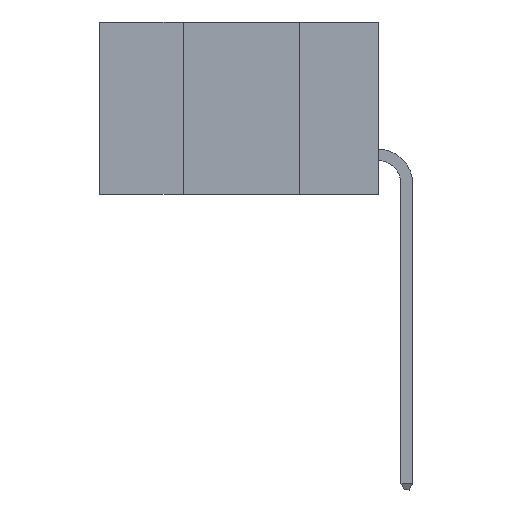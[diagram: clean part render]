
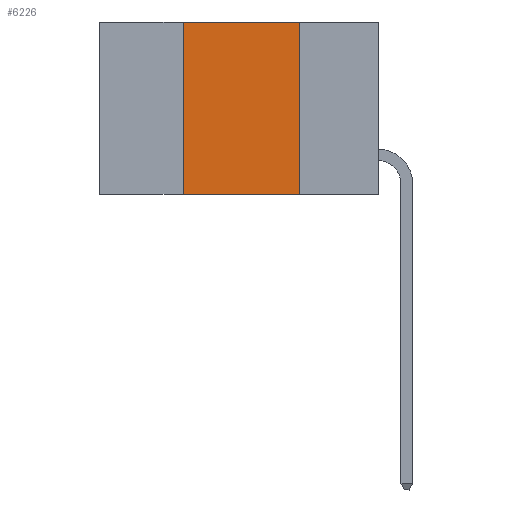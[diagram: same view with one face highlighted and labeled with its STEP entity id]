
A CAD part, left-side view. The second image highlights one B-rep face of the part: STEP entity #6226.
In plain terms, the highlighted planar face has unit normal (-1, 0, 0).
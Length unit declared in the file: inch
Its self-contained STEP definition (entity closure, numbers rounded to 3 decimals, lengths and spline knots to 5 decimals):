
#64 = LINE ( 'NONE', #14693, #9832 ) ;
#316 = CARTESIAN_POINT ( 'NONE',  ( 0., 0.6, 0. ) ) ;
#456 = ORIENTED_EDGE ( 'NONE', *, *, #13074, .F. ) ;
#1563 = EDGE_CURVE ( 'NONE', #14412, #10503, #13665, .T. ) ;
#2437 = DIRECTION ( 'NONE',  ( 1., 0., 0. ) ) ;
#2866 = VECTOR ( 'NONE', #14048, 39.37008 ) ;
#3201 = EDGE_LOOP ( 'NONE', ( #456, #20381, #21014, #17597 ) ) ;
#4754 = CARTESIAN_POINT ( 'NONE',  ( 0., 0.6, -0.37 ) ) ;
#6226 = ADVANCED_FACE ( 'NONE', ( #21511 ), #25641, .F. ) ;
#6513 = DIRECTION ( 'NONE',  ( 0., 0., -1. ) ) ;
#6536 = EDGE_CURVE ( 'NONE', #14412, #11100, #27109, .T. ) ;
#6825 = VECTOR ( 'NONE', #13027, 39.37008 ) ;
#7648 = LINE ( 'NONE', #10973, #20463 ) ;
#9028 = CARTESIAN_POINT ( 'NONE',  ( 0., 0.42, 0. ) ) ;
#9703 = AXIS2_PLACEMENT_3D ( 'NONE', #316, #2437, #6513 ) ;
#9832 = VECTOR ( 'NONE', #14422, 39.37008 ) ;
#10503 = VERTEX_POINT ( 'NONE', #14590 ) ;
#10973 = CARTESIAN_POINT ( 'NONE',  ( 0., 0.6, 0. ) ) ;
#11100 = VERTEX_POINT ( 'NONE', #9028 ) ;
#13027 = DIRECTION ( 'NONE',  ( 0., -1., 0. ) ) ;
#13074 = EDGE_CURVE ( 'NONE', #25797, #10503, #64, .T. ) ;
#13665 = LINE ( 'NONE', #4754, #6825 ) ;
#14048 = DIRECTION ( 'NONE',  ( 0., 0., 1. ) ) ;
#14412 = VERTEX_POINT ( 'NONE', #23943 ) ;
#14422 = DIRECTION ( 'NONE',  ( 0., 0., -1. ) ) ;
#14590 = CARTESIAN_POINT ( 'NONE',  ( 0., 0.17, -0.37 ) ) ;
#14693 = CARTESIAN_POINT ( 'NONE',  ( 0., 0.17, 0. ) ) ;
#17597 = ORIENTED_EDGE ( 'NONE', *, *, #1563, .T. ) ;
#20381 = ORIENTED_EDGE ( 'NONE', *, *, #26890, .F. ) ;
#20463 = VECTOR ( 'NONE', #21188, 39.37008 ) ;
#21014 = ORIENTED_EDGE ( 'NONE', *, *, #6536, .F. ) ;
#21188 = DIRECTION ( 'NONE',  ( 0., -1., 0. ) ) ;
#21511 = FACE_OUTER_BOUND ( 'NONE', #3201, .T. ) ;
#23943 = CARTESIAN_POINT ( 'NONE',  ( 0., 0.42, -0.37 ) ) ;
#24255 = CARTESIAN_POINT ( 'NONE',  ( 0., 0.17, 0. ) ) ;
#24516 = CARTESIAN_POINT ( 'NONE',  ( 0., 0.42, 0. ) ) ;
#25641 = PLANE ( 'NONE',  #9703 ) ;
#25797 = VERTEX_POINT ( 'NONE', #24255 ) ;
#26890 = EDGE_CURVE ( 'NONE', #11100, #25797, #7648, .T. ) ;
#27109 = LINE ( 'NONE', #24516, #2866 ) ;
